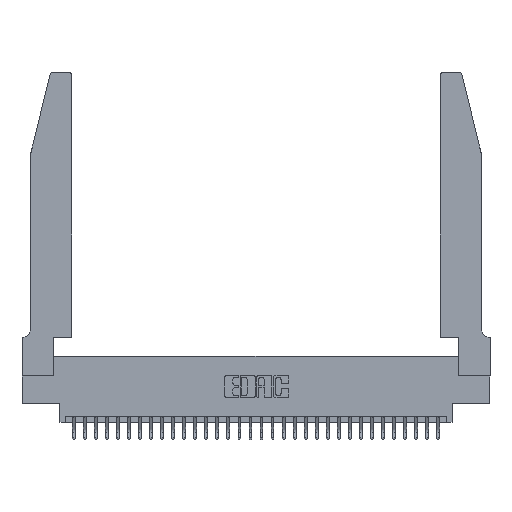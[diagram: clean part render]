
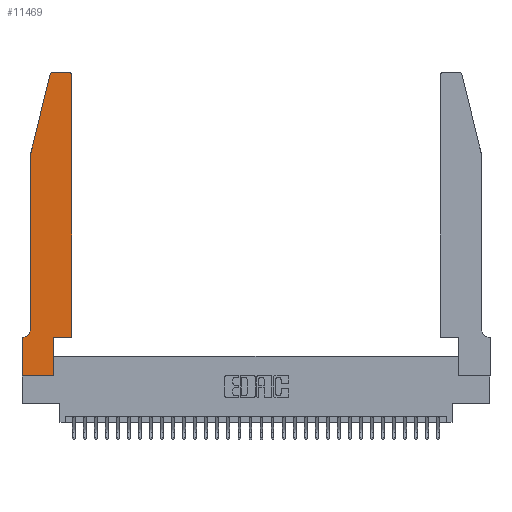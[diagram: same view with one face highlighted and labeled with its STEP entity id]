
A CAD part, top view. The second image highlights one B-rep face of the part: STEP entity #11469.
In plain terms, the highlighted planar face has unit normal (0, 0, 1).
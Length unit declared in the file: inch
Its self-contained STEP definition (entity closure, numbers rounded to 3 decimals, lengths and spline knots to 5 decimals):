
#119 = CARTESIAN_POINT ( 'NONE',  ( 0.0055, 0.35, 0.37 ) ) ;
#551 = ORIENTED_EDGE ( 'NONE', *, *, #16451, .T. ) ;
#955 = LINE ( 'NONE', #7678, #32722 ) ;
#1042 = AXIS2_PLACEMENT_3D ( 'NONE', #25908, #5577, #2921 ) ;
#1612 = VECTOR ( 'NONE', #5113, 39.37008 ) ;
#2112 = CARTESIAN_POINT ( 'NONE',  ( 0.4505, 0.35, 0.37 ) ) ;
#2148 = ORIENTED_EDGE ( 'NONE', *, *, #19679, .T. ) ;
#2327 = VERTEX_POINT ( 'NONE', #24721 ) ;
#2485 = LINE ( 'NONE', #7643, #3671 ) ;
#2683 = DIRECTION ( 'NONE',  ( 0., 1., 0. ) ) ;
#2754 = ORIENTED_EDGE ( 'NONE', *, *, #19384, .T. ) ;
#2761 = VERTEX_POINT ( 'NONE', #13838 ) ;
#2921 = DIRECTION ( 'NONE',  ( -1., 0., 0. ) ) ;
#3274 = VECTOR ( 'NONE', #30949, 39.37008 ) ;
#3671 = VECTOR ( 'NONE', #15668, 39.37008 ) ;
#4440 = LINE ( 'NONE', #23417, #3274 ) ;
#4658 = VERTEX_POINT ( 'NONE', #13954 ) ;
#4712 = CARTESIAN_POINT ( 'NONE',  ( 0.2865, 0.35, 0.37 ) ) ;
#4996 = VERTEX_POINT ( 'NONE', #13670 ) ;
#5113 = DIRECTION ( 'NONE',  ( -1., 0., 0. ) ) ;
#5457 = CARTESIAN_POINT ( 'NONE',  ( 0., 0., 0.37 ) ) ;
#5577 = DIRECTION ( 'NONE',  ( 0., 0., -1. ) ) ;
#5769 = DIRECTION ( 'NONE',  ( 1., 0., 0. ) ) ;
#6007 = LINE ( 'NONE', #20374, #29817 ) ;
#6097 = CARTESIAN_POINT ( 'NONE',  ( 0.284, 2.72, 0.37 ) ) ;
#6119 = EDGE_CURVE ( 'NONE', #21604, #20483, #6007, .T. ) ;
#6174 = VERTEX_POINT ( 'NONE', #22931 ) ;
#6884 = EDGE_CURVE ( 'NONE', #2327, #21604, #32573, .T. ) ;
#7220 = VECTOR ( 'NONE', #25794, 39.37008 ) ;
#7242 = DIRECTION ( 'NONE',  ( -0.239, -0.971, 0. ) ) ;
#7643 = CARTESIAN_POINT ( 'NONE',  ( 0.0755, 2., 0.37 ) ) ;
#7678 = CARTESIAN_POINT ( 'NONE',  ( 0.4505, 0.35, 0.37 ) ) ;
#7866 = DIRECTION ( 'NONE',  ( 1., 0., 0. ) ) ;
#8407 = FACE_OUTER_BOUND ( 'NONE', #18124, .T. ) ;
#9315 = CARTESIAN_POINT ( 'NONE',  ( 0., 0., 0.37 ) ) ;
#9523 = CARTESIAN_POINT ( 'NONE',  ( 0.4205, 2.72, 0.37 ) ) ;
#10165 = ORIENTED_EDGE ( 'NONE', *, *, #6119, .T. ) ;
#11469 = ADVANCED_FACE ( 'NONE', ( #8407 ), #23196, .T. ) ;
#11730 = AXIS2_PLACEMENT_3D ( 'NONE', #9523, #29423, #11987 ) ;
#11987 = DIRECTION ( 'NONE',  ( 1., 0., 0. ) ) ;
#13349 = DIRECTION ( 'NONE',  ( 0., 1., 0. ) ) ;
#13670 = CARTESIAN_POINT ( 'NONE',  ( 0.0755, 2., 0.37 ) ) ;
#13838 = CARTESIAN_POINT ( 'NONE',  ( 0.25487, 2.72718, 0.37 ) ) ;
#13954 = CARTESIAN_POINT ( 'NONE',  ( 0., 0.35, 0.37 ) ) ;
#13974 = ORIENTED_EDGE ( 'NONE', *, *, #18869, .T. ) ;
#14077 = ORIENTED_EDGE ( 'NONE', *, *, #6884, .T. ) ;
#14592 = EDGE_CURVE ( 'NONE', #15944, #2761, #27643, .T. ) ;
#15668 = DIRECTION ( 'NONE',  ( 0., -1., 0. ) ) ;
#15917 = EDGE_CURVE ( 'NONE', #18565, #17838, #19625, .T. ) ;
#15944 = VERTEX_POINT ( 'NONE', #28358 ) ;
#16241 = ORIENTED_EDGE ( 'NONE', *, *, #25879, .T. ) ;
#16294 = CARTESIAN_POINT ( 'NONE',  ( 0.0755, 0.42, 0.37 ) ) ;
#16451 = EDGE_CURVE ( 'NONE', #4996, #18565, #2485, .T. ) ;
#17748 = VECTOR ( 'NONE', #30668, 39.37008 ) ;
#17838 = VERTEX_POINT ( 'NONE', #119 ) ;
#18124 = EDGE_LOOP ( 'NONE', ( #19936, #21751, #13974, #551, #19694, #26193, #2148, #16241, #14077, #10165, #27975, #2754 ) ) ;
#18129 = DIRECTION ( 'NONE',  ( 1., 0., 0. ) ) ;
#18430 = CARTESIAN_POINT ( 'NONE',  ( 0.2605, 2.75, 0.37 ) ) ;
#18565 = VERTEX_POINT ( 'NONE', #16294 ) ;
#18869 = EDGE_CURVE ( 'NONE', #2761, #4996, #19955, .T. ) ;
#19325 = CARTESIAN_POINT ( 'NONE',  ( 0.4505, 2.72, 0.37 ) ) ;
#19349 = VERTEX_POINT ( 'NONE', #9315 ) ;
#19384 = EDGE_CURVE ( 'NONE', #20363, #6174, #20771, .T. ) ;
#19578 = VECTOR ( 'NONE', #7242, 39.37008 ) ;
#19625 = CIRCLE ( 'NONE', #1042, 0.07 ) ;
#19679 = EDGE_CURVE ( 'NONE', #4658, #19349, #4440, .T. ) ;
#19694 = ORIENTED_EDGE ( 'NONE', *, *, #15917, .T. ) ;
#19936 = ORIENTED_EDGE ( 'NONE', *, *, #29638, .T. ) ;
#19955 = LINE ( 'NONE', #29784, #19578 ) ;
#20363 = VERTEX_POINT ( 'NONE', #19325 ) ;
#20374 = CARTESIAN_POINT ( 'NONE',  ( 0.4505, 0.35, 0.37 ) ) ;
#20483 = VERTEX_POINT ( 'NONE', #2112 ) ;
#20529 = CARTESIAN_POINT ( 'NONE',  ( 0., 0.35, 0.37 ) ) ;
#20555 = EDGE_CURVE ( 'NONE', #17838, #4658, #29047, .T. ) ;
#20771 = CIRCLE ( 'NONE', #11730, 0.03 ) ;
#20858 = DIRECTION ( 'NONE',  ( 0., 0., 1. ) ) ;
#20972 = DIRECTION ( 'NONE',  ( 0., 0., 1. ) ) ;
#21444 = VECTOR ( 'NONE', #13349, 39.37008 ) ;
#21604 = VERTEX_POINT ( 'NONE', #4712 ) ;
#21751 = ORIENTED_EDGE ( 'NONE', *, *, #14592, .T. ) ;
#22111 = LINE ( 'NONE', #18430, #17748 ) ;
#22551 = CARTESIAN_POINT ( 'NONE',  ( 0.0755, 0.35, 0.37 ) ) ;
#22931 = CARTESIAN_POINT ( 'NONE',  ( 0.4205, 2.75, 0.37 ) ) ;
#23196 = PLANE ( 'NONE',  #26478 ) ;
#23329 = CARTESIAN_POINT ( 'NONE',  ( 0.2865, 0.35, 0.37 ) ) ;
#23417 = CARTESIAN_POINT ( 'NONE',  ( 0., 0., 0.37 ) ) ;
#24292 = LINE ( 'NONE', #5457, #7220 ) ;
#24721 = CARTESIAN_POINT ( 'NONE',  ( 0.2865, 0., 0.37 ) ) ;
#24742 = EDGE_CURVE ( 'NONE', #20483, #20363, #955, .T. ) ;
#25794 = DIRECTION ( 'NONE',  ( 1., 0., 0. ) ) ;
#25879 = EDGE_CURVE ( 'NONE', #19349, #2327, #24292, .T. ) ;
#25908 = CARTESIAN_POINT ( 'NONE',  ( 0.0055, 0.42, 0.37 ) ) ;
#26193 = ORIENTED_EDGE ( 'NONE', *, *, #20555, .T. ) ;
#26478 = AXIS2_PLACEMENT_3D ( 'NONE', #20529, #20858, #7866 ) ;
#27643 = CIRCLE ( 'NONE', #31424, 0.03 ) ;
#27975 = ORIENTED_EDGE ( 'NONE', *, *, #24742, .T. ) ;
#28358 = CARTESIAN_POINT ( 'NONE',  ( 0.284, 2.75, 0.37 ) ) ;
#29047 = LINE ( 'NONE', #22551, #1612 ) ;
#29423 = DIRECTION ( 'NONE',  ( 0., 0., 1. ) ) ;
#29638 = EDGE_CURVE ( 'NONE', #6174, #15944, #22111, .T. ) ;
#29784 = CARTESIAN_POINT ( 'NONE',  ( 0.0755, 2., 0.37 ) ) ;
#29817 = VECTOR ( 'NONE', #18129, 39.37008 ) ;
#30668 = DIRECTION ( 'NONE',  ( -1., 0., 0. ) ) ;
#30949 = DIRECTION ( 'NONE',  ( 0., -1., 0. ) ) ;
#31424 = AXIS2_PLACEMENT_3D ( 'NONE', #6097, #20972, #5769 ) ;
#32573 = LINE ( 'NONE', #23329, #21444 ) ;
#32722 = VECTOR ( 'NONE', #2683, 39.37008 ) ;
